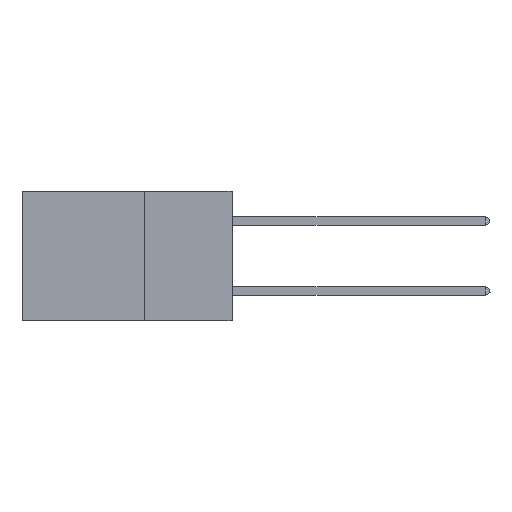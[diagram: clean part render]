
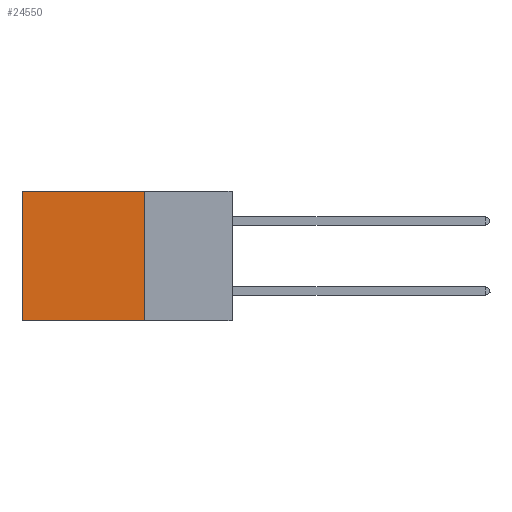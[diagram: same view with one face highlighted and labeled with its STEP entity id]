
A CAD part, left-side view. The second image highlights one B-rep face of the part: STEP entity #24550.
In plain terms, the highlighted planar face has unit normal (-1, 0, 0).
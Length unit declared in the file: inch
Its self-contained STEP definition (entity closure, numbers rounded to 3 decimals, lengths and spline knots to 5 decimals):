
#1247 = DIRECTION ( 'NONE',  ( 0., 1., 0. ) ) ;
#4116 = DIRECTION ( 'NONE',  ( 0., 0., -1. ) ) ;
#5034 = ORIENTED_EDGE ( 'NONE', *, *, #30400, .F. ) ;
#6569 = EDGE_CURVE ( 'NONE', #28910, #16102, #20682, .T. ) ;
#7926 = CARTESIAN_POINT ( 'NONE',  ( 0.2875, 0.25, 0. ) ) ;
#12981 = DIRECTION ( 'NONE',  ( 0., 0., -1. ) ) ;
#13375 = ORIENTED_EDGE ( 'NONE', *, *, #6569, .T. ) ;
#15882 = EDGE_CURVE ( 'NONE', #28685, #16102, #43310, .T. ) ;
#16102 = VERTEX_POINT ( 'NONE', #26158 ) ;
#16314 = DIRECTION ( 'NONE',  ( 1., 0., 0. ) ) ;
#17630 = LINE ( 'NONE', #41697, #36487 ) ;
#18237 = FACE_OUTER_BOUND ( 'NONE', #29437, .T. ) ;
#18382 = CARTESIAN_POINT ( 'NONE',  ( 0.2875, 0.25, -0.37 ) ) ;
#18396 = AXIS2_PLACEMENT_3D ( 'NONE', #43754, #16314, #12981 ) ;
#19106 = ORIENTED_EDGE ( 'NONE', *, *, #15882, .F. ) ;
#20682 = LINE ( 'NONE', #24784, #21783 ) ;
#21783 = VECTOR ( 'NONE', #4116, 39.37008 ) ;
#22255 = ORIENTED_EDGE ( 'NONE', *, *, #40218, .T. ) ;
#23574 = VERTEX_POINT ( 'NONE', #7926 ) ;
#24550 = ADVANCED_FACE ( 'NONE', ( #18237 ), #37127, .F. ) ;
#24784 = CARTESIAN_POINT ( 'NONE',  ( 0.2875, 0.6, 0. ) ) ;
#26037 = LINE ( 'NONE', #42379, #43299 ) ;
#26158 = CARTESIAN_POINT ( 'NONE',  ( 0.2875, 0.6, -0.37 ) ) ;
#27850 = DIRECTION ( 'NONE',  ( 0., 1., 0. ) ) ;
#28685 = VERTEX_POINT ( 'NONE', #18382 ) ;
#28910 = VERTEX_POINT ( 'NONE', #29709 ) ;
#29437 = EDGE_LOOP ( 'NONE', ( #13375, #19106, #5034, #22255 ) ) ;
#29709 = CARTESIAN_POINT ( 'NONE',  ( 0.2875, 0.6, 0. ) ) ;
#30375 = VECTOR ( 'NONE', #1247, 39.37008 ) ;
#30400 = EDGE_CURVE ( 'NONE', #23574, #28685, #26037, .T. ) ;
#31858 = DIRECTION ( 'NONE',  ( 0., 0., -1. ) ) ;
#35814 = CARTESIAN_POINT ( 'NONE',  ( 0.2875, 0.25, -0.37 ) ) ;
#36487 = VECTOR ( 'NONE', #27850, 39.37008 ) ;
#37127 = PLANE ( 'NONE',  #18396 ) ;
#40218 = EDGE_CURVE ( 'NONE', #23574, #28910, #17630, .T. ) ;
#41697 = CARTESIAN_POINT ( 'NONE',  ( 0.2875, 0.25, 0. ) ) ;
#42379 = CARTESIAN_POINT ( 'NONE',  ( 0.2875, 0.25, 0. ) ) ;
#43299 = VECTOR ( 'NONE', #31858, 39.37008 ) ;
#43310 = LINE ( 'NONE', #35814, #30375 ) ;
#43754 = CARTESIAN_POINT ( 'NONE',  ( 0.2875, 0.25, 0. ) ) ;
